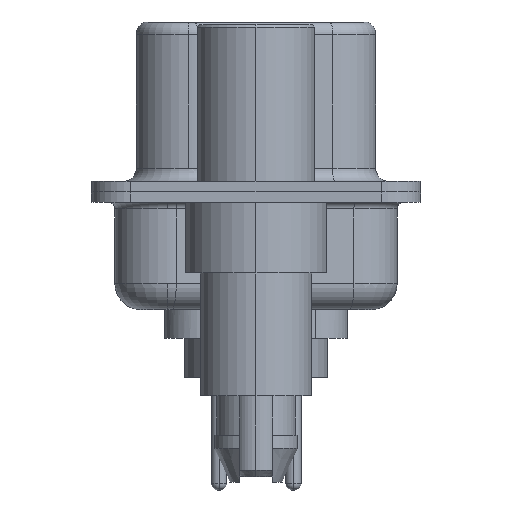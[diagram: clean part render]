
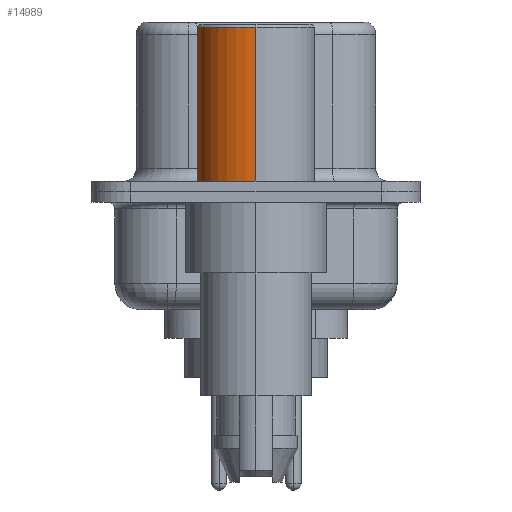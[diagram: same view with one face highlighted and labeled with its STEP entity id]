
A CAD part, left-side view. The second image highlights one B-rep face of the part: STEP entity #14989.
In plain terms, the highlighted cylindrical face has radius 2.25 mm (diameter 4.5 mm), a partial arc.
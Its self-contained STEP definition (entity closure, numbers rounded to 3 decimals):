
#298 = EDGE_CURVE ( 'NONE', #14117, #15551, #19103, .T. ) ;
#800 = AXIS2_PLACEMENT_3D ( 'NONE', #3577, #15370, #5309 ) ;
#2174 = VECTOR ( 'NONE', #15338, 1000. ) ;
#2436 = AXIS2_PLACEMENT_3D ( 'NONE', #17471, #9087, #20866 ) ;
#2535 = EDGE_CURVE ( 'NONE', #14117, #15207, #12166, .T. ) ;
#2893 = EDGE_LOOP ( 'NONE', ( #16647, #21712, #18668, #16220 ) ) ;
#3551 = CARTESIAN_POINT ( 'NONE',  ( -2.25, 0., 0.581 ) ) ;
#3577 = CARTESIAN_POINT ( 'NONE',  ( 0., 0., 6.3 ) ) ;
#3927 = DIRECTION ( 'NONE',  ( 0., 0., 1. ) ) ;
#4393 = AXIS2_PLACEMENT_3D ( 'NONE', #7140, #18919, #8829 ) ;
#4988 = CYLINDRICAL_SURFACE ( 'NONE', #2436, 2.25 ) ;
#5131 = VECTOR ( 'NONE', #3927, 1000. ) ;
#5309 = DIRECTION ( 'NONE',  ( 1., 0., 0. ) ) ;
#5641 = CARTESIAN_POINT ( 'NONE',  ( 2.25, 0., 0.581 ) ) ;
#7140 = CARTESIAN_POINT ( 'NONE',  ( 0., 0., 0.4 ) ) ;
#7860 = VERTEX_POINT ( 'NONE', #15934 ) ;
#7889 = CARTESIAN_POINT ( 'NONE',  ( -2.25, 0., 0.4 ) ) ;
#7965 = CIRCLE ( 'NONE', #800, 2.25 ) ;
#8829 = DIRECTION ( 'NONE',  ( 1., 0., 0. ) ) ;
#8984 = EDGE_CURVE ( 'NONE', #15551, #7860, #7965, .T. ) ;
#9087 = DIRECTION ( 'NONE',  ( 0., 0., 1. ) ) ;
#10012 = FACE_OUTER_BOUND ( 'NONE', #2893, .T. ) ;
#10075 = CARTESIAN_POINT ( 'NONE',  ( 2.25, 0., 0.4 ) ) ;
#12166 = CIRCLE ( 'NONE', #4393, 2.25 ) ;
#13745 = CARTESIAN_POINT ( 'NONE',  ( 2.25, 0., 6.3 ) ) ;
#14117 = VERTEX_POINT ( 'NONE', #10075 ) ;
#14989 = ADVANCED_FACE ( 'NONE', ( #10012 ), #4988, .T. ) ;
#15207 = VERTEX_POINT ( 'NONE', #7889 ) ;
#15338 = DIRECTION ( 'NONE',  ( 0., 0., 1. ) ) ;
#15370 = DIRECTION ( 'NONE',  ( 0., 0., 1. ) ) ;
#15551 = VERTEX_POINT ( 'NONE', #13745 ) ;
#15934 = CARTESIAN_POINT ( 'NONE',  ( -2.25, 0., 6.3 ) ) ;
#16220 = ORIENTED_EDGE ( 'NONE', *, *, #298, .F. ) ;
#16647 = ORIENTED_EDGE ( 'NONE', *, *, #2535, .T. ) ;
#17471 = CARTESIAN_POINT ( 'NONE',  ( 0., 0., 0.581 ) ) ;
#18668 = ORIENTED_EDGE ( 'NONE', *, *, #8984, .F. ) ;
#18919 = DIRECTION ( 'NONE',  ( 0., 0., 1. ) ) ;
#19103 = LINE ( 'NONE', #5641, #5131 ) ;
#19525 = LINE ( 'NONE', #3551, #2174 ) ;
#20457 = EDGE_CURVE ( 'NONE', #15207, #7860, #19525, .T. ) ;
#20866 = DIRECTION ( 'NONE',  ( 1., 0., 0. ) ) ;
#21712 = ORIENTED_EDGE ( 'NONE', *, *, #20457, .T. ) ;
